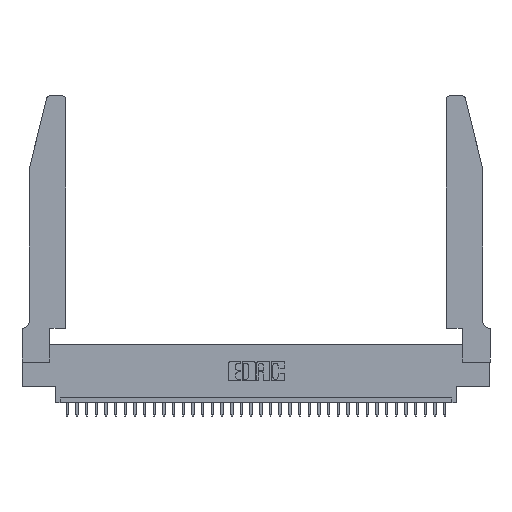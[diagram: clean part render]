
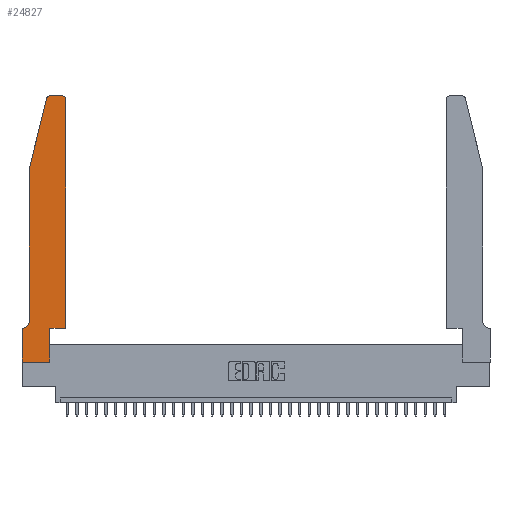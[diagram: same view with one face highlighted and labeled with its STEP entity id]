
A CAD part, top view. The second image highlights one B-rep face of the part: STEP entity #24827.
In plain terms, the highlighted planar face has unit normal (0, 0, 1).
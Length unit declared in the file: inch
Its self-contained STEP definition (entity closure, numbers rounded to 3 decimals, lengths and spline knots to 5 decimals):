
#198 = CARTESIAN_POINT ( 'NONE',  ( 0.2865, 0.35, 0.37 ) ) ;
#272 = CARTESIAN_POINT ( 'NONE',  ( 0.4505, 0.35, 0.37 ) ) ;
#498 = EDGE_CURVE ( 'NONE', #28718, #1458, #35159, .T. ) ;
#692 = VECTOR ( 'NONE', #11461, 39.37008 ) ;
#1089 = VERTEX_POINT ( 'NONE', #7571 ) ;
#1090 = CARTESIAN_POINT ( 'NONE',  ( 0.4205, 2.72, 0.37 ) ) ;
#1189 = EDGE_CURVE ( 'NONE', #29741, #3926, #28291, .T. ) ;
#1376 = AXIS2_PLACEMENT_3D ( 'NONE', #1090, #22978, #14823 ) ;
#1458 = VERTEX_POINT ( 'NONE', #17853 ) ;
#1568 = EDGE_CURVE ( 'NONE', #18944, #13336, #25709, .T. ) ;
#1741 = VECTOR ( 'NONE', #8760, 39.37008 ) ;
#2404 = DIRECTION ( 'NONE',  ( 0., -1., 0. ) ) ;
#2716 = DIRECTION ( 'NONE',  ( -0.239, -0.971, 0. ) ) ;
#2900 = CARTESIAN_POINT ( 'NONE',  ( 0.0755, 2., 0.37 ) ) ;
#3154 = VERTEX_POINT ( 'NONE', #21962 ) ;
#3580 = FACE_OUTER_BOUND ( 'NONE', #21198, .T. ) ;
#3918 = CARTESIAN_POINT ( 'NONE',  ( 0.0755, 0.42, 0.37 ) ) ;
#3926 = VERTEX_POINT ( 'NONE', #13127 ) ;
#4269 = PLANE ( 'NONE',  #18658 ) ;
#4382 = DIRECTION ( 'NONE',  ( 0., 0., 1. ) ) ;
#4898 = VECTOR ( 'NONE', #24657, 39.37008 ) ;
#5120 = AXIS2_PLACEMENT_3D ( 'NONE', #28292, #20224, #17127 ) ;
#5969 = ORIENTED_EDGE ( 'NONE', *, *, #20271, .T. ) ;
#6207 = DIRECTION ( 'NONE',  ( -1., 0., 0. ) ) ;
#6238 = EDGE_CURVE ( 'NONE', #3154, #19396, #32315, .T. ) ;
#7017 = CARTESIAN_POINT ( 'NONE',  ( 0.2865, 0.35, 0.37 ) ) ;
#7280 = LINE ( 'NONE', #26936, #1741 ) ;
#7571 = CARTESIAN_POINT ( 'NONE',  ( 0.2865, 0., 0.37 ) ) ;
#8089 = CARTESIAN_POINT ( 'NONE',  ( 0.2605, 2.75, 0.37 ) ) ;
#8638 = LINE ( 'NONE', #31178, #15488 ) ;
#8760 = DIRECTION ( 'NONE',  ( 1., 0., 0. ) ) ;
#8782 = EDGE_CURVE ( 'NONE', #1089, #16592, #13438, .T. ) ;
#9053 = DIRECTION ( 'NONE',  ( 0., 0., -1. ) ) ;
#9599 = CARTESIAN_POINT ( 'NONE',  ( 0.25487, 2.72718, 0.37 ) ) ;
#9656 = DIRECTION ( 'NONE',  ( 1., 0., 0. ) ) ;
#10369 = EDGE_CURVE ( 'NONE', #12039, #18944, #15048, .T. ) ;
#10881 = EDGE_CURVE ( 'NONE', #13336, #30434, #34136, .T. ) ;
#10933 = ORIENTED_EDGE ( 'NONE', *, *, #1189, .T. ) ;
#11122 = VECTOR ( 'NONE', #2404, 39.37008 ) ;
#11461 = DIRECTION ( 'NONE',  ( 0., 1., 0. ) ) ;
#11910 = ORIENTED_EDGE ( 'NONE', *, *, #6238, .T. ) ;
#12039 = VERTEX_POINT ( 'NONE', #3918 ) ;
#13127 = CARTESIAN_POINT ( 'NONE',  ( 0.0755, 2., 0.37 ) ) ;
#13336 = VERTEX_POINT ( 'NONE', #19864 ) ;
#13438 = LINE ( 'NONE', #198, #4898 ) ;
#13604 = AXIS2_PLACEMENT_3D ( 'NONE', #25311, #9053, #6207 ) ;
#14823 = DIRECTION ( 'NONE',  ( 1., 0., 0. ) ) ;
#15048 = CIRCLE ( 'NONE', #13604, 0.07 ) ;
#15244 = LINE ( 'NONE', #2900, #25779 ) ;
#15417 = CARTESIAN_POINT ( 'NONE',  ( 0.4505, 0.35, 0.37 ) ) ;
#15488 = VECTOR ( 'NONE', #9656, 39.37008 ) ;
#15663 = ORIENTED_EDGE ( 'NONE', *, *, #18169, .T. ) ;
#16385 = VECTOR ( 'NONE', #22215, 39.37008 ) ;
#16592 = VERTEX_POINT ( 'NONE', #7017 ) ;
#17127 = DIRECTION ( 'NONE',  ( 1., 0., 0. ) ) ;
#17853 = CARTESIAN_POINT ( 'NONE',  ( 0.4505, 2.72, 0.37 ) ) ;
#18169 = EDGE_CURVE ( 'NONE', #19396, #29741, #21400, .T. ) ;
#18239 = ORIENTED_EDGE ( 'NONE', *, *, #10369, .T. ) ;
#18425 = EDGE_CURVE ( 'NONE', #16592, #28718, #8638, .T. ) ;
#18658 = AXIS2_PLACEMENT_3D ( 'NONE', #34493, #4382, #20680 ) ;
#18944 = VERTEX_POINT ( 'NONE', #19565 ) ;
#19017 = CARTESIAN_POINT ( 'NONE',  ( 0.0755, 2., 0.37 ) ) ;
#19396 = VERTEX_POINT ( 'NONE', #28201 ) ;
#19565 = CARTESIAN_POINT ( 'NONE',  ( 0.0055, 0.35, 0.37 ) ) ;
#19716 = ORIENTED_EDGE ( 'NONE', *, *, #1568, .T. ) ;
#19864 = CARTESIAN_POINT ( 'NONE',  ( 0., 0.35, 0.37 ) ) ;
#20224 = DIRECTION ( 'NONE',  ( 0., 0., 1. ) ) ;
#20271 = EDGE_CURVE ( 'NONE', #30434, #1089, #7280, .T. ) ;
#20530 = CIRCLE ( 'NONE', #1376, 0.03 ) ;
#20680 = DIRECTION ( 'NONE',  ( 1., 0., 0. ) ) ;
#21198 = EDGE_LOOP ( 'NONE', ( #11910, #15663, #10933, #25391, #18239, #19716, #23974, #5969, #31753, #29436, #27138, #25778 ) ) ;
#21400 = CIRCLE ( 'NONE', #5120, 0.03 ) ;
#21962 = CARTESIAN_POINT ( 'NONE',  ( 0.4205, 2.75, 0.37 ) ) ;
#22215 = DIRECTION ( 'NONE',  ( -1., 0., 0. ) ) ;
#22483 = VECTOR ( 'NONE', #32833, 39.37008 ) ;
#22978 = DIRECTION ( 'NONE',  ( 0., 0., 1. ) ) ;
#23329 = EDGE_CURVE ( 'NONE', #3926, #12039, #15244, .T. ) ;
#23974 = ORIENTED_EDGE ( 'NONE', *, *, #10881, .T. ) ;
#24657 = DIRECTION ( 'NONE',  ( 0., 1., 0. ) ) ;
#24827 = ADVANCED_FACE ( 'NONE', ( #3580 ), #4269, .T. ) ;
#25311 = CARTESIAN_POINT ( 'NONE',  ( 0.0055, 0.42, 0.37 ) ) ;
#25391 = ORIENTED_EDGE ( 'NONE', *, *, #23329, .T. ) ;
#25709 = LINE ( 'NONE', #30287, #16385 ) ;
#25778 = ORIENTED_EDGE ( 'NONE', *, *, #26489, .T. ) ;
#25779 = VECTOR ( 'NONE', #30374, 39.37008 ) ;
#26489 = EDGE_CURVE ( 'NONE', #1458, #3154, #20530, .T. ) ;
#26936 = CARTESIAN_POINT ( 'NONE',  ( 0., 0., 0.37 ) ) ;
#27138 = ORIENTED_EDGE ( 'NONE', *, *, #498, .T. ) ;
#28201 = CARTESIAN_POINT ( 'NONE',  ( 0.284, 2.75, 0.37 ) ) ;
#28291 = LINE ( 'NONE', #19017, #29974 ) ;
#28292 = CARTESIAN_POINT ( 'NONE',  ( 0.284, 2.72, 0.37 ) ) ;
#28718 = VERTEX_POINT ( 'NONE', #15417 ) ;
#29436 = ORIENTED_EDGE ( 'NONE', *, *, #18425, .T. ) ;
#29741 = VERTEX_POINT ( 'NONE', #9599 ) ;
#29974 = VECTOR ( 'NONE', #2716, 39.37008 ) ;
#30104 = CARTESIAN_POINT ( 'NONE',  ( 0., 0., 0.37 ) ) ;
#30287 = CARTESIAN_POINT ( 'NONE',  ( 0.0755, 0.35, 0.37 ) ) ;
#30374 = DIRECTION ( 'NONE',  ( 0., -1., 0. ) ) ;
#30434 = VERTEX_POINT ( 'NONE', #30954 ) ;
#30954 = CARTESIAN_POINT ( 'NONE',  ( 0., 0., 0.37 ) ) ;
#31178 = CARTESIAN_POINT ( 'NONE',  ( 0.4505, 0.35, 0.37 ) ) ;
#31753 = ORIENTED_EDGE ( 'NONE', *, *, #8782, .T. ) ;
#32315 = LINE ( 'NONE', #8089, #22483 ) ;
#32833 = DIRECTION ( 'NONE',  ( -1., 0., 0. ) ) ;
#34136 = LINE ( 'NONE', #30104, #11122 ) ;
#34493 = CARTESIAN_POINT ( 'NONE',  ( 0., 0.35, 0.37 ) ) ;
#35159 = LINE ( 'NONE', #272, #692 ) ;
